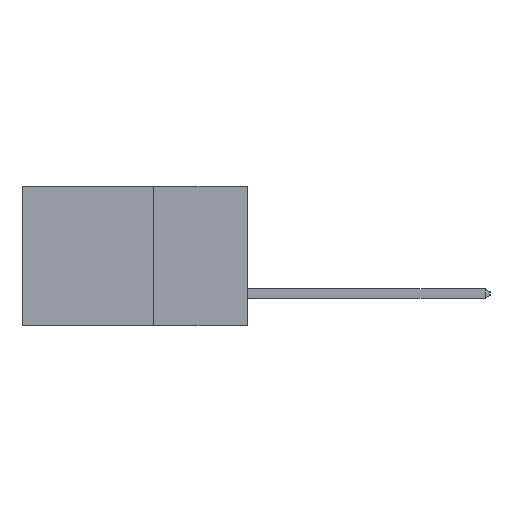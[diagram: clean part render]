
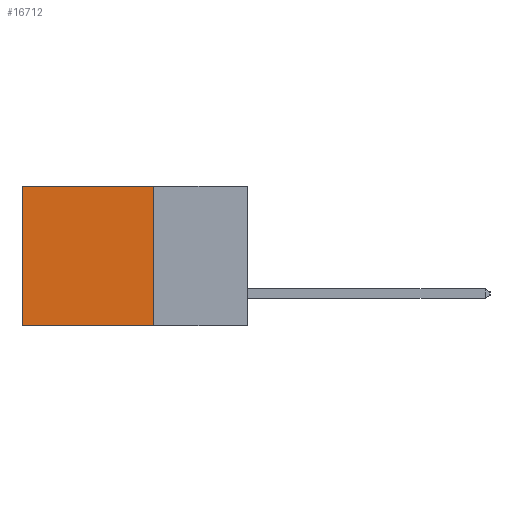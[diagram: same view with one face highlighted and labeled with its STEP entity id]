
A CAD part, left-side view. The second image highlights one B-rep face of the part: STEP entity #16712.
In plain terms, the highlighted planar face has unit normal (-1, 0, 0).
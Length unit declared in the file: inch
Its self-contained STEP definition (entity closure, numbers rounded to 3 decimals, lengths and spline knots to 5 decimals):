
#39 = CARTESIAN_POINT ( 'NONE',  ( 0.298, 0.25, -0.37 ) ) ;
#323 = EDGE_CURVE ( 'NONE', #17410, #13553, #13427, .T. ) ;
#1514 = CARTESIAN_POINT ( 'NONE',  ( 0.298, 0.25, 0. ) ) ;
#2594 = AXIS2_PLACEMENT_3D ( 'NONE', #1514, #17618, #8042 ) ;
#2711 = CARTESIAN_POINT ( 'NONE',  ( 0.298, 0.25, 0. ) ) ;
#2859 = FACE_OUTER_BOUND ( 'NONE', #19350, .T. ) ;
#3295 = DIRECTION ( 'NONE',  ( 0., 0., -1. ) ) ;
#4747 = DIRECTION ( 'NONE',  ( 0., 1., 0. ) ) ;
#5286 = EDGE_CURVE ( 'NONE', #13553, #16381, #10699, .T. ) ;
#5308 = VECTOR ( 'NONE', #3295, 39.37008 ) ;
#5888 = ORIENTED_EDGE ( 'NONE', *, *, #5286, .T. ) ;
#6402 = PLANE ( 'NONE',  #2594 ) ;
#8042 = DIRECTION ( 'NONE',  ( 0., 0., -1. ) ) ;
#8080 = DIRECTION ( 'NONE',  ( 0., 1., 0. ) ) ;
#8134 = VERTEX_POINT ( 'NONE', #39 ) ;
#8163 = EDGE_CURVE ( 'NONE', #8134, #16381, #17112, .T. ) ;
#10699 = LINE ( 'NONE', #20712, #5308 ) ;
#12480 = DIRECTION ( 'NONE',  ( 0., 0., -1. ) ) ;
#12968 = VECTOR ( 'NONE', #4747, 39.37008 ) ;
#13106 = VECTOR ( 'NONE', #12480, 39.37008 ) ;
#13427 = LINE ( 'NONE', #17140, #17086 ) ;
#13553 = VERTEX_POINT ( 'NONE', #15974 ) ;
#13637 = ORIENTED_EDGE ( 'NONE', *, *, #8163, .F. ) ;
#14544 = CARTESIAN_POINT ( 'NONE',  ( 0.298, 0.25, 0. ) ) ;
#14645 = ORIENTED_EDGE ( 'NONE', *, *, #15810, .F. ) ;
#15810 = EDGE_CURVE ( 'NONE', #17410, #8134, #17247, .T. ) ;
#15974 = CARTESIAN_POINT ( 'NONE',  ( 0.298, 0.6, 0. ) ) ;
#16381 = VERTEX_POINT ( 'NONE', #18329 ) ;
#16712 = ADVANCED_FACE ( 'NONE', ( #2859 ), #6402, .F. ) ;
#17086 = VECTOR ( 'NONE', #8080, 39.37008 ) ;
#17112 = LINE ( 'NONE', #19522, #12968 ) ;
#17140 = CARTESIAN_POINT ( 'NONE',  ( 0.298, 0.25, 0. ) ) ;
#17247 = LINE ( 'NONE', #2711, #13106 ) ;
#17410 = VERTEX_POINT ( 'NONE', #14544 ) ;
#17618 = DIRECTION ( 'NONE',  ( 1., 0., 0. ) ) ;
#18329 = CARTESIAN_POINT ( 'NONE',  ( 0.298, 0.6, -0.37 ) ) ;
#19350 = EDGE_LOOP ( 'NONE', ( #5888, #13637, #14645, #19793 ) ) ;
#19522 = CARTESIAN_POINT ( 'NONE',  ( 0.298, 0.25, -0.37 ) ) ;
#19793 = ORIENTED_EDGE ( 'NONE', *, *, #323, .T. ) ;
#20712 = CARTESIAN_POINT ( 'NONE',  ( 0.298, 0.6, 0. ) ) ;
